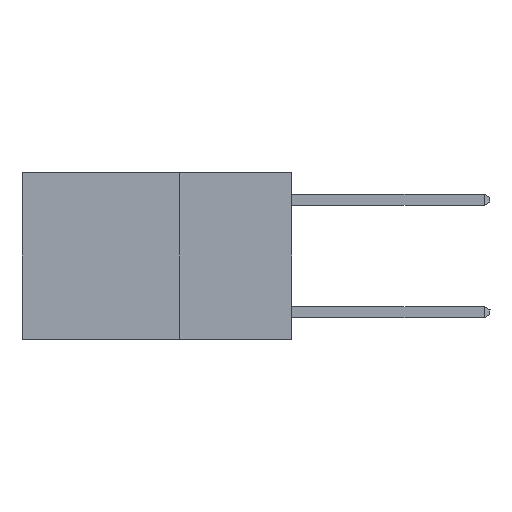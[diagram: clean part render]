
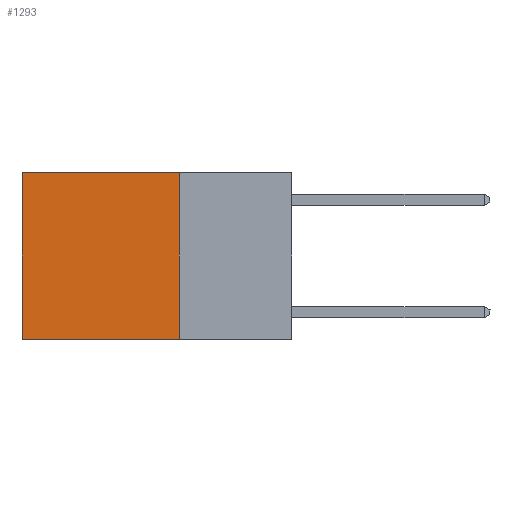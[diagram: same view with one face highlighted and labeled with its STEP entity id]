
A CAD part, left-side view. The second image highlights one B-rep face of the part: STEP entity #1293.
In plain terms, the highlighted planar face has unit normal (-1, 0, 0).
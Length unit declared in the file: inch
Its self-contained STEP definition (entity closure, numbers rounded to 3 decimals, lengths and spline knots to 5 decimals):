
#122 = EDGE_CURVE ( 'NONE', #8759, #9209, #1171, .T. ) ;
#468 = VERTEX_POINT ( 'NONE', #9672 ) ;
#1171 = LINE ( 'NONE', #15569, #12566 ) ;
#1293 = ADVANCED_FACE ( 'NONE', ( #7349 ), #3518, .F. ) ;
#1516 = DIRECTION ( 'NONE',  ( 0., 1., 0. ) ) ;
#2495 = EDGE_CURVE ( 'NONE', #468, #8759, #6511, .T. ) ;
#2593 = ORIENTED_EDGE ( 'NONE', *, *, #10133, .F. ) ;
#2693 = ORIENTED_EDGE ( 'NONE', *, *, #122, .T. ) ;
#2887 = LINE ( 'NONE', #4288, #5887 ) ;
#3017 = EDGE_CURVE ( 'NONE', #6666, #9209, #2887, .T. ) ;
#3518 = PLANE ( 'NONE',  #4728 ) ;
#3589 = VECTOR ( 'NONE', #15575, 39.37008 ) ;
#4260 = EDGE_LOOP ( 'NONE', ( #2693, #13005, #2593, #15328 ) ) ;
#4288 = CARTESIAN_POINT ( 'NONE',  ( 0.2625, 0.25, -0.37 ) ) ;
#4728 = AXIS2_PLACEMENT_3D ( 'NONE', #16428, #13752, #7273 ) ;
#5357 = CARTESIAN_POINT ( 'NONE',  ( 0.2625, 0.25, 0. ) ) ;
#5406 = LINE ( 'NONE', #5357, #3589 ) ;
#5887 = VECTOR ( 'NONE', #1516, 39.37008 ) ;
#6511 = LINE ( 'NONE', #12452, #7935 ) ;
#6666 = VERTEX_POINT ( 'NONE', #13982 ) ;
#6698 = CARTESIAN_POINT ( 'NONE',  ( 0.2625, 0.6, -0.37 ) ) ;
#7273 = DIRECTION ( 'NONE',  ( 0., 0., -1. ) ) ;
#7349 = FACE_OUTER_BOUND ( 'NONE', #4260, .T. ) ;
#7818 = DIRECTION ( 'NONE',  ( 0., 0., -1. ) ) ;
#7935 = VECTOR ( 'NONE', #11399, 39.37008 ) ;
#8759 = VERTEX_POINT ( 'NONE', #14760 ) ;
#9209 = VERTEX_POINT ( 'NONE', #6698 ) ;
#9672 = CARTESIAN_POINT ( 'NONE',  ( 0.2625, 0.25, 0. ) ) ;
#10133 = EDGE_CURVE ( 'NONE', #468, #6666, #5406, .T. ) ;
#11399 = DIRECTION ( 'NONE',  ( 0., 1., 0. ) ) ;
#12452 = CARTESIAN_POINT ( 'NONE',  ( 0.2625, 0.25, 0. ) ) ;
#12566 = VECTOR ( 'NONE', #7818, 39.37008 ) ;
#13005 = ORIENTED_EDGE ( 'NONE', *, *, #3017, .F. ) ;
#13752 = DIRECTION ( 'NONE',  ( 1., 0., 0. ) ) ;
#13982 = CARTESIAN_POINT ( 'NONE',  ( 0.2625, 0.25, -0.37 ) ) ;
#14760 = CARTESIAN_POINT ( 'NONE',  ( 0.2625, 0.6, 0. ) ) ;
#15328 = ORIENTED_EDGE ( 'NONE', *, *, #2495, .T. ) ;
#15569 = CARTESIAN_POINT ( 'NONE',  ( 0.2625, 0.6, 0. ) ) ;
#15575 = DIRECTION ( 'NONE',  ( 0., 0., -1. ) ) ;
#16428 = CARTESIAN_POINT ( 'NONE',  ( 0.2625, 0.25, 0. ) ) ;
